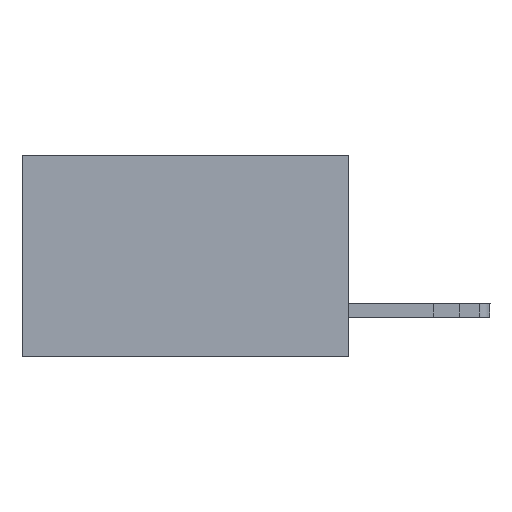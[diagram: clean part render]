
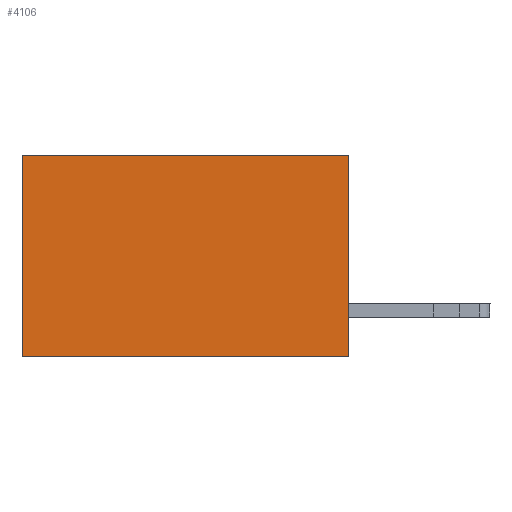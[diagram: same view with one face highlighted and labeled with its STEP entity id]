
A CAD part, left-side view. The second image highlights one B-rep face of the part: STEP entity #4106.
In plain terms, the highlighted planar face has unit normal (-1, 0, 0).
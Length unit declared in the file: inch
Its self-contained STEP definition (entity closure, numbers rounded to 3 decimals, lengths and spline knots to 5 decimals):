
#327 = LINE ( 'NONE', #5360, #18648 ) ;
#1572 = DIRECTION ( 'NONE',  ( 0., 1., 0. ) ) ;
#4106 = ADVANCED_FACE ( 'NONE', ( #20894 ), #16103, .F. ) ;
#4552 = VERTEX_POINT ( 'NONE', #6824 ) ;
#4912 = CARTESIAN_POINT ( 'NONE',  ( 0.2615, 0., -0.37 ) ) ;
#5123 = DIRECTION ( 'NONE',  ( 0., 0., -1. ) ) ;
#5360 = CARTESIAN_POINT ( 'NONE',  ( 0.2615, 0., 0. ) ) ;
#5642 = ORIENTED_EDGE ( 'NONE', *, *, #15661, .T. ) ;
#5929 = CARTESIAN_POINT ( 'NONE',  ( 0.2615, 0.6, -0.37 ) ) ;
#6761 = VECTOR ( 'NONE', #1572, 39.37008 ) ;
#6824 = CARTESIAN_POINT ( 'NONE',  ( 0.2615, 0.6, 0. ) ) ;
#7632 = CARTESIAN_POINT ( 'NONE',  ( 0.2615, 0., -0.37 ) ) ;
#8467 = LINE ( 'NONE', #11502, #18968 ) ;
#8607 = ORIENTED_EDGE ( 'NONE', *, *, #16459, .T. ) ;
#8684 = VERTEX_POINT ( 'NONE', #5929 ) ;
#9737 = LINE ( 'NONE', #18089, #6761 ) ;
#9756 = CARTESIAN_POINT ( 'NONE',  ( 0.2615, 0., -0.37 ) ) ;
#11502 = CARTESIAN_POINT ( 'NONE',  ( 0.2615, 0.6, -0.37 ) ) ;
#12567 = ORIENTED_EDGE ( 'NONE', *, *, #17010, .F. ) ;
#13440 = VERTEX_POINT ( 'NONE', #19518 ) ;
#13601 = EDGE_CURVE ( 'NONE', #17444, #8684, #9737, .T. ) ;
#14307 = AXIS2_PLACEMENT_3D ( 'NONE', #7632, #21212, #17931 ) ;
#14917 = DIRECTION ( 'NONE',  ( 0., 1., 0. ) ) ;
#15102 = DIRECTION ( 'NONE',  ( 0., 0., -1. ) ) ;
#15661 = EDGE_CURVE ( 'NONE', #4552, #8684, #8467, .T. ) ;
#16103 = PLANE ( 'NONE',  #14307 ) ;
#16459 = EDGE_CURVE ( 'NONE', #13440, #4552, #327, .T. ) ;
#17010 = EDGE_CURVE ( 'NONE', #13440, #17444, #19772, .T. ) ;
#17444 = VERTEX_POINT ( 'NONE', #9756 ) ;
#17931 = DIRECTION ( 'NONE',  ( 0., 0., -1. ) ) ;
#18089 = CARTESIAN_POINT ( 'NONE',  ( 0.2615, 0., -0.37 ) ) ;
#18648 = VECTOR ( 'NONE', #14917, 39.37008 ) ;
#18968 = VECTOR ( 'NONE', #15102, 39.37008 ) ;
#19518 = CARTESIAN_POINT ( 'NONE',  ( 0.2615, 0., 0. ) ) ;
#19715 = EDGE_LOOP ( 'NONE', ( #5642, #19989, #12567, #8607 ) ) ;
#19772 = LINE ( 'NONE', #4912, #20711 ) ;
#19989 = ORIENTED_EDGE ( 'NONE', *, *, #13601, .F. ) ;
#20711 = VECTOR ( 'NONE', #5123, 39.37008 ) ;
#20894 = FACE_OUTER_BOUND ( 'NONE', #19715, .T. ) ;
#21212 = DIRECTION ( 'NONE',  ( 1., 0., 0. ) ) ;
